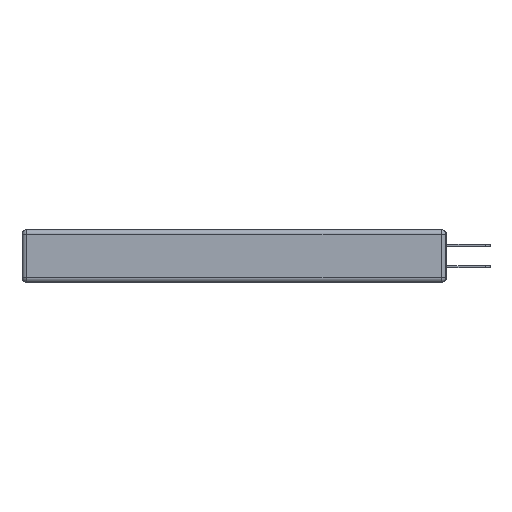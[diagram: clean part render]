
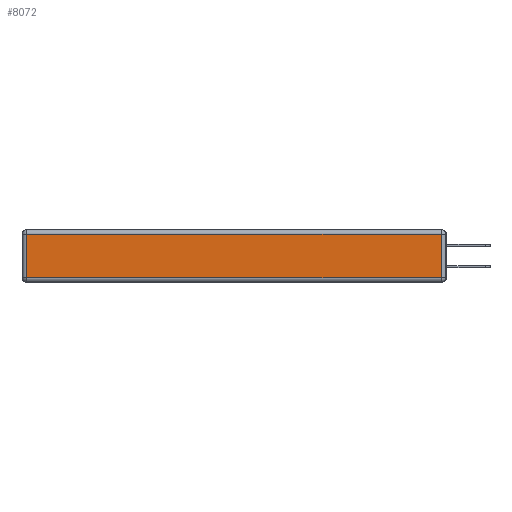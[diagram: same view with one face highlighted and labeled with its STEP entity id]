
A CAD part, left-side view. The second image highlights one B-rep face of the part: STEP entity #8072.
In plain terms, the highlighted planar face has unit normal (-1, 0, 0).
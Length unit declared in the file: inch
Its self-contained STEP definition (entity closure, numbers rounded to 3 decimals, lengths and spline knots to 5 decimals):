
#872 = EDGE_CURVE ( 'NONE', #28673, #4930, #7019, .T. ) ;
#2222 = ORIENTED_EDGE ( 'NONE', *, *, #872, .T. ) ;
#2821 = CARTESIAN_POINT ( 'NONE',  ( 0., 0.03, -0.343 ) ) ;
#4104 = AXIS2_PLACEMENT_3D ( 'NONE', #25229, #14702, #27601 ) ;
#4930 = VERTEX_POINT ( 'NONE', #16463 ) ;
#5255 = VECTOR ( 'NONE', #20302, 39.37008 ) ;
#6546 = CARTESIAN_POINT ( 'NONE',  ( 0., 0.03, -0.03 ) ) ;
#7019 = LINE ( 'NONE', #19704, #5255 ) ;
#8072 = ADVANCED_FACE ( 'NONE', ( #21043 ), #14229, .T. ) ;
#9316 = EDGE_LOOP ( 'NONE', ( #2222, #16978, #18391, #16651 ) ) ;
#11562 = EDGE_CURVE ( 'NONE', #18277, #15953, #14248, .T. ) ;
#12741 = EDGE_CURVE ( 'NONE', #4930, #18277, #18677, .T. ) ;
#13293 = DIRECTION ( 'NONE',  ( 0., 0., -1. ) ) ;
#13924 = CARTESIAN_POINT ( 'NONE',  ( 0., 2.72, -0.03 ) ) ;
#14229 = PLANE ( 'NONE',  #4104 ) ;
#14248 = LINE ( 'NONE', #18513, #19468 ) ;
#14702 = DIRECTION ( 'NONE',  ( -1., 0., 0. ) ) ;
#15953 = VERTEX_POINT ( 'NONE', #13924 ) ;
#16046 = DIRECTION ( 'NONE',  ( 0., 0., 1. ) ) ;
#16463 = CARTESIAN_POINT ( 'NONE',  ( 0., 0.03, -0.313 ) ) ;
#16651 = ORIENTED_EDGE ( 'NONE', *, *, #18832, .T. ) ;
#16978 = ORIENTED_EDGE ( 'NONE', *, *, #12741, .T. ) ;
#18277 = VERTEX_POINT ( 'NONE', #6546 ) ;
#18391 = ORIENTED_EDGE ( 'NONE', *, *, #11562, .T. ) ;
#18403 = LINE ( 'NONE', #24706, #26420 ) ;
#18513 = CARTESIAN_POINT ( 'NONE',  ( 0., 2.75, -0.03 ) ) ;
#18677 = LINE ( 'NONE', #2821, #23220 ) ;
#18832 = EDGE_CURVE ( 'NONE', #15953, #28673, #18403, .T. ) ;
#19468 = VECTOR ( 'NONE', #23094, 39.37008 ) ;
#19704 = CARTESIAN_POINT ( 'NONE',  ( 0., 0., -0.313 ) ) ;
#20302 = DIRECTION ( 'NONE',  ( 0., -1., 0. ) ) ;
#21043 = FACE_OUTER_BOUND ( 'NONE', #9316, .T. ) ;
#23094 = DIRECTION ( 'NONE',  ( 0., 1., 0. ) ) ;
#23220 = VECTOR ( 'NONE', #16046, 39.37008 ) ;
#24568 = CARTESIAN_POINT ( 'NONE',  ( 0., 2.72, -0.313 ) ) ;
#24706 = CARTESIAN_POINT ( 'NONE',  ( 0., 2.72, -0.343 ) ) ;
#25229 = CARTESIAN_POINT ( 'NONE',  ( 0., 0., -0.343 ) ) ;
#26420 = VECTOR ( 'NONE', #13293, 39.37008 ) ;
#27601 = DIRECTION ( 'NONE',  ( 0., 0., 1. ) ) ;
#28673 = VERTEX_POINT ( 'NONE', #24568 ) ;
